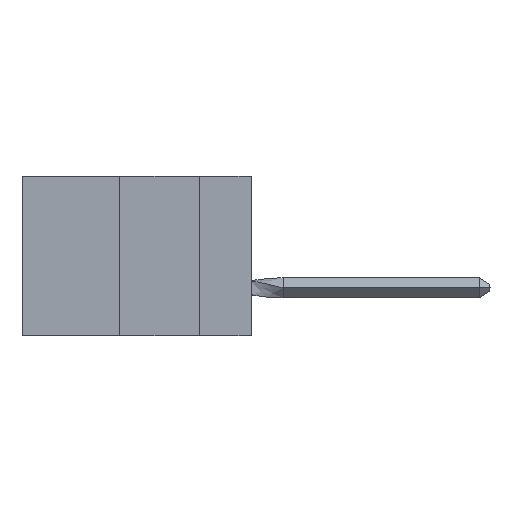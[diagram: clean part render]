
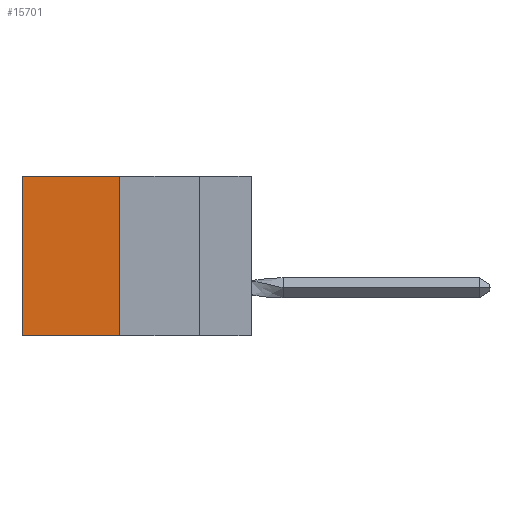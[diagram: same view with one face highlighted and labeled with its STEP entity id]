
A CAD part, left-side view. The second image highlights one B-rep face of the part: STEP entity #15701.
In plain terms, the highlighted planar face has unit normal (-1, 0, 0).
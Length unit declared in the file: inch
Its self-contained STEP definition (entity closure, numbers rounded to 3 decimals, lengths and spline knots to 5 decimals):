
#438 = DIRECTION ( 'NONE',  ( 0., 0., -1. ) ) ;
#560 = FACE_OUTER_BOUND ( 'NONE', #9222, .T. ) ;
#1553 = ORIENTED_EDGE ( 'NONE', *, *, #12689, .T. ) ;
#2217 = CARTESIAN_POINT ( 'NONE',  ( 0.305, 0.413, -0.5 ) ) ;
#2313 = VECTOR ( 'NONE', #438, 39.37008 ) ;
#2601 = PLANE ( 'NONE',  #6178 ) ;
#2675 = CARTESIAN_POINT ( 'NONE',  ( 0.305, 0.413, 0. ) ) ;
#3459 = CARTESIAN_POINT ( 'NONE',  ( 0.305, 0.413, 0. ) ) ;
#3706 = ORIENTED_EDGE ( 'NONE', *, *, #3764, .F. ) ;
#3764 = EDGE_CURVE ( 'NONE', #14641, #4344, #5255, .T. ) ;
#4344 = VERTEX_POINT ( 'NONE', #8201 ) ;
#4655 = DIRECTION ( 'NONE',  ( 0., 0., -1. ) ) ;
#5255 = LINE ( 'NONE', #2217, #6227 ) ;
#5472 = LINE ( 'NONE', #3459, #6091 ) ;
#5572 = ORIENTED_EDGE ( 'NONE', *, *, #7964, .T. ) ;
#6091 = VECTOR ( 'NONE', #14649, 39.37008 ) ;
#6178 = AXIS2_PLACEMENT_3D ( 'NONE', #8715, #11431, #6217 ) ;
#6217 = DIRECTION ( 'NONE',  ( 0., 0., -1. ) ) ;
#6227 = VECTOR ( 'NONE', #12283, 39.37008 ) ;
#6961 = CARTESIAN_POINT ( 'NONE',  ( 0.305, 0.72, -0.5 ) ) ;
#7213 = ORIENTED_EDGE ( 'NONE', *, *, #10890, .F. ) ;
#7964 = EDGE_CURVE ( 'NONE', #13493, #4344, #10378, .T. ) ;
#8201 = CARTESIAN_POINT ( 'NONE',  ( 0.305, 0.72, -0.5 ) ) ;
#8715 = CARTESIAN_POINT ( 'NONE',  ( 0.305, 0.413, -0.5 ) ) ;
#9222 = EDGE_LOOP ( 'NONE', ( #5572, #3706, #7213, #1553 ) ) ;
#9898 = CARTESIAN_POINT ( 'NONE',  ( 0.305, 0.72, 0. ) ) ;
#10378 = LINE ( 'NONE', #6961, #2313 ) ;
#10453 = CARTESIAN_POINT ( 'NONE',  ( 0.305, 0.413, -0.5 ) ) ;
#10890 = EDGE_CURVE ( 'NONE', #15145, #14641, #15601, .T. ) ;
#11431 = DIRECTION ( 'NONE',  ( 1., 0., 0. ) ) ;
#11682 = VECTOR ( 'NONE', #4655, 39.37008 ) ;
#12283 = DIRECTION ( 'NONE',  ( 0., 1., 0. ) ) ;
#12689 = EDGE_CURVE ( 'NONE', #15145, #13493, #5472, .T. ) ;
#13493 = VERTEX_POINT ( 'NONE', #9898 ) ;
#14634 = CARTESIAN_POINT ( 'NONE',  ( 0.305, 0.413, -0.5 ) ) ;
#14641 = VERTEX_POINT ( 'NONE', #10453 ) ;
#14649 = DIRECTION ( 'NONE',  ( 0., 1., 0. ) ) ;
#15145 = VERTEX_POINT ( 'NONE', #2675 ) ;
#15601 = LINE ( 'NONE', #14634, #11682 ) ;
#15701 = ADVANCED_FACE ( 'NONE', ( #560 ), #2601, .F. ) ;
